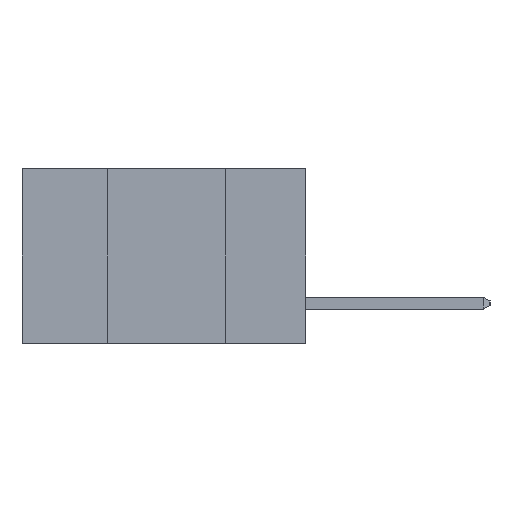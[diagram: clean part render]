
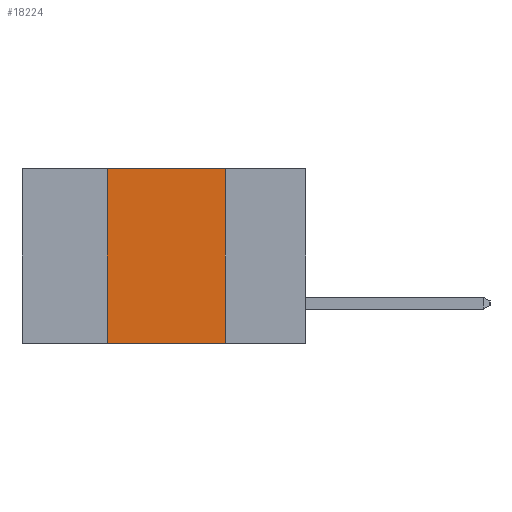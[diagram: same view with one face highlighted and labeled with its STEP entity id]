
A CAD part, left-side view. The second image highlights one B-rep face of the part: STEP entity #18224.
In plain terms, the highlighted planar face has unit normal (-1, 0, 0).
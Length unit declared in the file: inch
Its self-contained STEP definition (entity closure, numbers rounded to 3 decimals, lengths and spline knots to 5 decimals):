
#737 = VERTEX_POINT ( 'NONE', #14025 ) ;
#1082 = DIRECTION ( 'NONE',  ( 1., 0., 0. ) ) ;
#1147 = DIRECTION ( 'NONE',  ( 0., -1., 0. ) ) ;
#1733 = CARTESIAN_POINT ( 'NONE',  ( 0., 0.6, -0.37 ) ) ;
#2653 = VERTEX_POINT ( 'NONE', #13903 ) ;
#2924 = VECTOR ( 'NONE', #17694, 39.37008 ) ;
#2963 = EDGE_LOOP ( 'NONE', ( #6177, #8363, #10221, #7260 ) ) ;
#5073 = CARTESIAN_POINT ( 'NONE',  ( 0., 0.42, 0. ) ) ;
#5336 = VECTOR ( 'NONE', #5867, 39.37008 ) ;
#5726 = EDGE_CURVE ( 'NONE', #17089, #2653, #9848, .T. ) ;
#5867 = DIRECTION ( 'NONE',  ( 0., -1., 0. ) ) ;
#5934 = CARTESIAN_POINT ( 'NONE',  ( 0., 0.6, 0. ) ) ;
#5996 = VECTOR ( 'NONE', #1147, 39.37008 ) ;
#6177 = ORIENTED_EDGE ( 'NONE', *, *, #17998, .F. ) ;
#6740 = EDGE_CURVE ( 'NONE', #17089, #18335, #7897, .T. ) ;
#6904 = DIRECTION ( 'NONE',  ( 0., 0., 1. ) ) ;
#7260 = ORIENTED_EDGE ( 'NONE', *, *, #5726, .T. ) ;
#7897 = LINE ( 'NONE', #5073, #11609 ) ;
#7952 = CARTESIAN_POINT ( 'NONE',  ( 0., 0.17, 0. ) ) ;
#8363 = ORIENTED_EDGE ( 'NONE', *, *, #14614, .F. ) ;
#9848 = LINE ( 'NONE', #1733, #5996 ) ;
#10061 = CARTESIAN_POINT ( 'NONE',  ( 0., 0.42, 0. ) ) ;
#10221 = ORIENTED_EDGE ( 'NONE', *, *, #6740, .F. ) ;
#11184 = DIRECTION ( 'NONE',  ( 0., 0., -1. ) ) ;
#11609 = VECTOR ( 'NONE', #6904, 39.37008 ) ;
#12890 = LINE ( 'NONE', #5934, #5336 ) ;
#13614 = FACE_OUTER_BOUND ( 'NONE', #2963, .T. ) ;
#13903 = CARTESIAN_POINT ( 'NONE',  ( 0., 0.17, -0.37 ) ) ;
#13949 = CARTESIAN_POINT ( 'NONE',  ( 0., 0.6, 0. ) ) ;
#14025 = CARTESIAN_POINT ( 'NONE',  ( 0., 0.17, 0. ) ) ;
#14246 = CARTESIAN_POINT ( 'NONE',  ( 0., 0.42, -0.37 ) ) ;
#14614 = EDGE_CURVE ( 'NONE', #18335, #737, #12890, .T. ) ;
#14788 = AXIS2_PLACEMENT_3D ( 'NONE', #13949, #1082, #11184 ) ;
#16754 = PLANE ( 'NONE',  #14788 ) ;
#17089 = VERTEX_POINT ( 'NONE', #14246 ) ;
#17524 = LINE ( 'NONE', #7952, #2924 ) ;
#17694 = DIRECTION ( 'NONE',  ( 0., 0., -1. ) ) ;
#17998 = EDGE_CURVE ( 'NONE', #737, #2653, #17524, .T. ) ;
#18224 = ADVANCED_FACE ( 'NONE', ( #13614 ), #16754, .F. ) ;
#18335 = VERTEX_POINT ( 'NONE', #10061 ) ;
